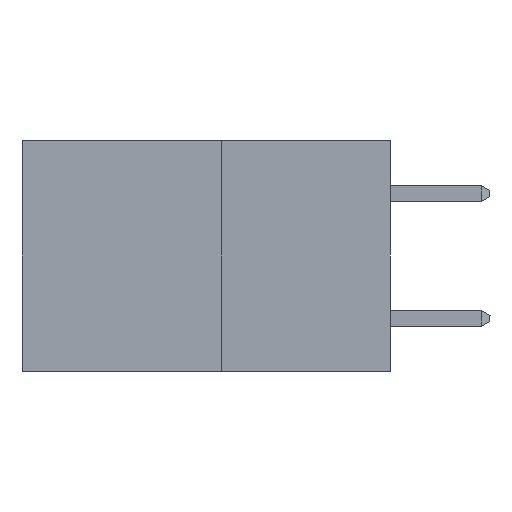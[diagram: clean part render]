
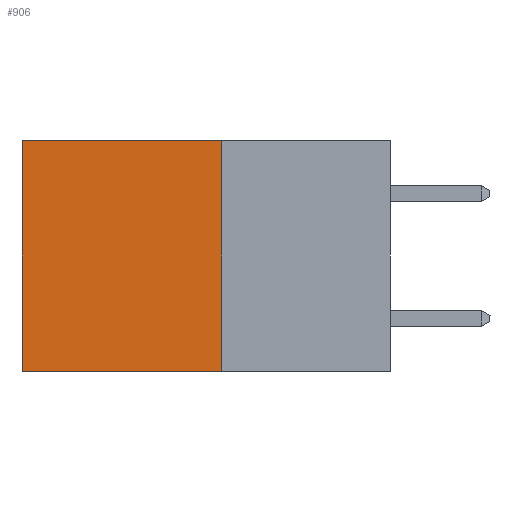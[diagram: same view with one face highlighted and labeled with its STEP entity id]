
A CAD part, left-side view. The second image highlights one B-rep face of the part: STEP entity #906.
In plain terms, the highlighted planar face has unit normal (-1, 0, 0).
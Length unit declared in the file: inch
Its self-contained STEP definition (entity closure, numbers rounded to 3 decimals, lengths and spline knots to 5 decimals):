
#1 = EDGE_CURVE ( 'NONE', #6889, #7160, #8661, .T. ) ;
#78 = ORIENTED_EDGE ( 'NONE', *, *, #3669, .T. ) ;
#180 = VERTEX_POINT ( 'NONE', #1598 ) ;
#709 = DIRECTION ( 'NONE',  ( 0., 0., -1. ) ) ;
#760 = CARTESIAN_POINT ( 'NONE',  ( 0.277, 0.59, -0.37 ) ) ;
#906 = ADVANCED_FACE ( 'NONE', ( #2867 ), #7508, .F. ) ;
#1002 = ORIENTED_EDGE ( 'NONE', *, *, #1, .F. ) ;
#1082 = EDGE_LOOP ( 'NONE', ( #1594, #1380, #1002, #78 ) ) ;
#1380 = ORIENTED_EDGE ( 'NONE', *, *, #7662, .F. ) ;
#1443 = VECTOR ( 'NONE', #8172, 39.37008 ) ;
#1594 = ORIENTED_EDGE ( 'NONE', *, *, #8709, .T. ) ;
#1598 = CARTESIAN_POINT ( 'NONE',  ( 0.277, 0.59, 0. ) ) ;
#1652 = AXIS2_PLACEMENT_3D ( 'NONE', #7213, #7263, #8269 ) ;
#2170 = CARTESIAN_POINT ( 'NONE',  ( 0.277, 0.27, -0.37 ) ) ;
#2867 = FACE_OUTER_BOUND ( 'NONE', #1082, .T. ) ;
#3269 = LINE ( 'NONE', #6820, #1443 ) ;
#3669 = EDGE_CURVE ( 'NONE', #6889, #180, #3269, .T. ) ;
#4750 = CARTESIAN_POINT ( 'NONE',  ( 0.277, 0.27, -0.37 ) ) ;
#5685 = CARTESIAN_POINT ( 'NONE',  ( 0.277, 0.27, 0. ) ) ;
#6363 = VECTOR ( 'NONE', #709, 39.37008 ) ;
#6754 = VECTOR ( 'NONE', #8139, 39.37008 ) ;
#6820 = CARTESIAN_POINT ( 'NONE',  ( 0.277, 0.27, 0. ) ) ;
#6889 = VERTEX_POINT ( 'NONE', #5685 ) ;
#7160 = VERTEX_POINT ( 'NONE', #4750 ) ;
#7213 = CARTESIAN_POINT ( 'NONE',  ( 0.277, 0.27, -0.37 ) ) ;
#7263 = DIRECTION ( 'NONE',  ( 1., 0., 0. ) ) ;
#7505 = VERTEX_POINT ( 'NONE', #760 ) ;
#7508 = PLANE ( 'NONE',  #1652 ) ;
#7628 = LINE ( 'NONE', #8786, #9306 ) ;
#7662 = EDGE_CURVE ( 'NONE', #7160, #7505, #7628, .T. ) ;
#8139 = DIRECTION ( 'NONE',  ( 0., 0., -1. ) ) ;
#8172 = DIRECTION ( 'NONE',  ( 0., 1., 0. ) ) ;
#8269 = DIRECTION ( 'NONE',  ( 0., 0., -1. ) ) ;
#8283 = LINE ( 'NONE', #8909, #6363 ) ;
#8661 = LINE ( 'NONE', #2170, #6754 ) ;
#8692 = DIRECTION ( 'NONE',  ( 0., 1., 0. ) ) ;
#8709 = EDGE_CURVE ( 'NONE', #180, #7505, #8283, .T. ) ;
#8786 = CARTESIAN_POINT ( 'NONE',  ( 0.277, 0.27, -0.37 ) ) ;
#8909 = CARTESIAN_POINT ( 'NONE',  ( 0.277, 0.59, -0.37 ) ) ;
#9306 = VECTOR ( 'NONE', #8692, 39.37008 ) ;
